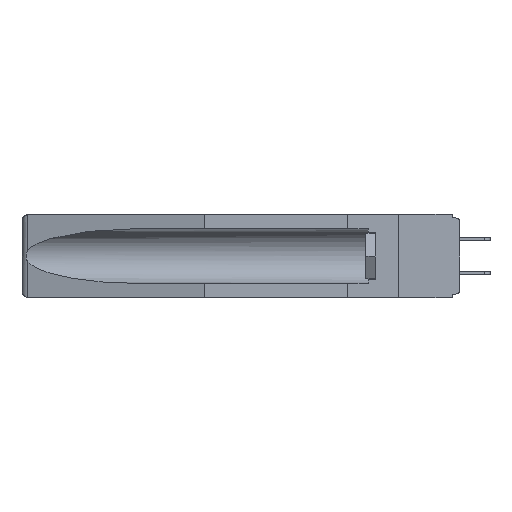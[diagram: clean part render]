
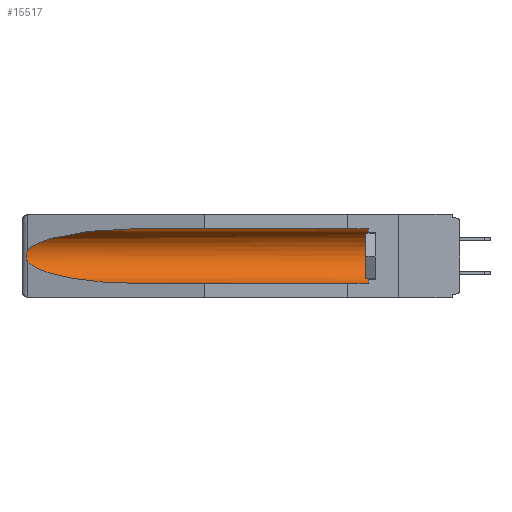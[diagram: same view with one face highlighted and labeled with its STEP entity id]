
A CAD part, left-side view. The second image highlights one B-rep face of the part: STEP entity #15517.
In plain terms, the highlighted cylindrical face has radius 2.857 mm (diameter 5.715 mm), a partial arc.
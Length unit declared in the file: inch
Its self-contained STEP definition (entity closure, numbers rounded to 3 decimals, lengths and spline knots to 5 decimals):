
#765 = DIRECTION ( 'NONE',  ( 0., 1., 0. ) ) ;
#938 = CIRCLE ( 'NONE', #21683, 0.1125 ) ;
#1346 =( BOUNDED_CURVE ( )  B_SPLINE_CURVE ( 3, ( #20767, #8707, #5745, #20909 ),
 .UNSPECIFIED., .F., .F. ) 
 B_SPLINE_CURVE_WITH_KNOTS ( ( 4, 4 ),
 ( 0.1948, 1.5708 ),
 .UNSPECIFIED. ) 
 CURVE ( )  GEOMETRIC_REPRESENTATION_ITEM ( )  RATIONAL_B_SPLINE_CURVE ( ( 1., 0.848, 0.848, 1. ) ) 
 REPRESENTATION_ITEM ( '' )  );
#1363 = VERTEX_POINT ( 'NONE', #11344 ) ;
#1572 = CARTESIAN_POINT ( 'NONE',  ( 0.2673, 1.53269, -0.17917 ) ) ;
#2002 = VERTEX_POINT ( 'NONE', #14145 ) ;
#2487 = DIRECTION ( 'NONE',  ( 0., 0., 1. ) ) ;
#2609 = ORIENTED_EDGE ( 'NONE', *, *, #9027, .F. ) ;
#2702 = EDGE_CURVE ( 'NONE', #5412, #9034, #938, .T. ) ;
#2891 = ORIENTED_EDGE ( 'NONE', *, *, #17941, .T. ) ;
#3269 = CARTESIAN_POINT ( 'NONE',  ( 0.26537, 1.52718, -0.19328 ) ) ;
#3649 =( BOUNDED_CURVE ( )  B_SPLINE_CURVE ( 3, ( #18236, #14746, #11474, #13053 ),
 .UNSPECIFIED., .F., .F. ) 
 B_SPLINE_CURVE_WITH_KNOTS ( ( 4, 4 ),
 ( 4.71239, 6.08839 ),
 .UNSPECIFIED. ) 
 CURVE ( )  GEOMETRIC_REPRESENTATION_ITEM ( )  RATIONAL_B_SPLINE_CURVE ( ( 1., 0.848, 0.848, 1. ) ) 
 REPRESENTATION_ITEM ( '' )  );
#4111 = CARTESIAN_POINT ( 'NONE',  ( 0.26537, 1.52718, -0.19328 ) ) ;
#4586 = B_SPLINE_CURVE_WITH_KNOTS ( 'NONE', 3,
 ( #11456, #16532, #21253, #6183, #9970, #11816, #1572, #13535, #13384, #3269 ),
 .UNSPECIFIED., .F., .F.,
 ( 4, 2, 2, 2, 4 ),
 ( 0., 0.00029, 0.00058, 0.00087, 0.00117 ),
 .UNSPECIFIED. ) ;
#4861 = CARTESIAN_POINT ( 'NONE',  ( 0.26537, 1.52718, -0.14972 ) ) ;
#5291 = CARTESIAN_POINT ( 'NONE',  ( 0.155, -0.30754, -0.059 ) ) ;
#5412 = VERTEX_POINT ( 'NONE', #18108 ) ;
#5745 = CARTESIAN_POINT ( 'NONE',  ( 0.21114, 1.30732, -0.284 ) ) ;
#6183 = CARTESIAN_POINT ( 'NONE',  ( 0.2673, 1.5327, -0.16383 ) ) ;
#6345 = EDGE_CURVE ( 'NONE', #16460, #18060, #4586, .T. ) ;
#6752 = CARTESIAN_POINT ( 'NONE',  ( 0.155, 0.126, -0.1715 ) ) ;
#8429 = DIRECTION ( 'NONE',  ( 0., -1., 0. ) ) ;
#8707 = CARTESIAN_POINT ( 'NONE',  ( 0.25451, 1.48313, -0.24835 ) ) ;
#8734 = ORIENTED_EDGE ( 'NONE', *, *, #6345, .T. ) ;
#9027 = EDGE_CURVE ( 'NONE', #5412, #1363, #21311, .T. ) ;
#9034 = VERTEX_POINT ( 'NONE', #16307 ) ;
#9229 = ORIENTED_EDGE ( 'NONE', *, *, #2702, .T. ) ;
#9970 = CARTESIAN_POINT ( 'NONE',  ( 0.2675, 1.53308, -0.16763 ) ) ;
#10734 = EDGE_LOOP ( 'NONE', ( #17557, #8734, #11190, #2609, #9229, #2891 ) ) ;
#10834 = FACE_OUTER_BOUND ( 'NONE', #10734, .T. ) ;
#11098 = CARTESIAN_POINT ( 'NONE',  ( 0.155, -0.30754, -0.1715 ) ) ;
#11190 = ORIENTED_EDGE ( 'NONE', *, *, #15924, .T. ) ;
#11344 = CARTESIAN_POINT ( 'NONE',  ( 0.155, 1.07973, -0.284 ) ) ;
#11456 = CARTESIAN_POINT ( 'NONE',  ( 0.26537, 1.52718, -0.14972 ) ) ;
#11474 = CARTESIAN_POINT ( 'NONE',  ( 0.25451, 1.48313, -0.09465 ) ) ;
#11816 = CARTESIAN_POINT ( 'NONE',  ( 0.2675, 1.53308, -0.17534 ) ) ;
#11877 = VECTOR ( 'NONE', #17071, 39.37008 ) ;
#13053 = CARTESIAN_POINT ( 'NONE',  ( 0.26537, 1.52718, -0.14972 ) ) ;
#13155 = EDGE_CURVE ( 'NONE', #2002, #16460, #3649, .T. ) ;
#13384 = CARTESIAN_POINT ( 'NONE',  ( 0.26597, 1.5296, -0.19026 ) ) ;
#13535 = CARTESIAN_POINT ( 'NONE',  ( 0.26655, 1.53094, -0.18657 ) ) ;
#14145 = CARTESIAN_POINT ( 'NONE',  ( 0.155, 1.07973, -0.059 ) ) ;
#14746 = CARTESIAN_POINT ( 'NONE',  ( 0.21114, 1.30732, -0.059 ) ) ;
#14813 = CYLINDRICAL_SURFACE ( 'NONE', #21421, 0.1125 ) ;
#14852 = CARTESIAN_POINT ( 'NONE',  ( 0.155, -0.30754, -0.284 ) ) ;
#15517 = ADVANCED_FACE ( 'NONE', ( #10834 ), #14813, .F. ) ;
#15924 = EDGE_CURVE ( 'NONE', #18060, #1363, #1346, .T. ) ;
#16118 = LINE ( 'NONE', #5291, #11877 ) ;
#16307 = CARTESIAN_POINT ( 'NONE',  ( 0.155, 0.126, -0.059 ) ) ;
#16460 = VERTEX_POINT ( 'NONE', #4861 ) ;
#16532 = CARTESIAN_POINT ( 'NONE',  ( 0.26597, 1.52961, -0.15275 ) ) ;
#17071 = DIRECTION ( 'NONE',  ( 0., 1., 0. ) ) ;
#17352 = VECTOR ( 'NONE', #18198, 39.37008 ) ;
#17557 = ORIENTED_EDGE ( 'NONE', *, *, #13155, .T. ) ;
#17941 = EDGE_CURVE ( 'NONE', #9034, #2002, #16118, .T. ) ;
#18060 = VERTEX_POINT ( 'NONE', #4111 ) ;
#18108 = CARTESIAN_POINT ( 'NONE',  ( 0.155, 0.126, -0.284 ) ) ;
#18198 = DIRECTION ( 'NONE',  ( 0., 1., 0. ) ) ;
#18236 = CARTESIAN_POINT ( 'NONE',  ( 0.155, 1.07973, -0.059 ) ) ;
#20186 = DIRECTION ( 'NONE',  ( 0., 0., 1. ) ) ;
#20767 = CARTESIAN_POINT ( 'NONE',  ( 0.26537, 1.52718, -0.19328 ) ) ;
#20909 = CARTESIAN_POINT ( 'NONE',  ( 0.155, 1.07973, -0.284 ) ) ;
#21253 = CARTESIAN_POINT ( 'NONE',  ( 0.26654, 1.53092, -0.15636 ) ) ;
#21311 = LINE ( 'NONE', #14852, #17352 ) ;
#21421 = AXIS2_PLACEMENT_3D ( 'NONE', #11098, #765, #2487 ) ;
#21683 = AXIS2_PLACEMENT_3D ( 'NONE', #6752, #8429, #20186 ) ;
